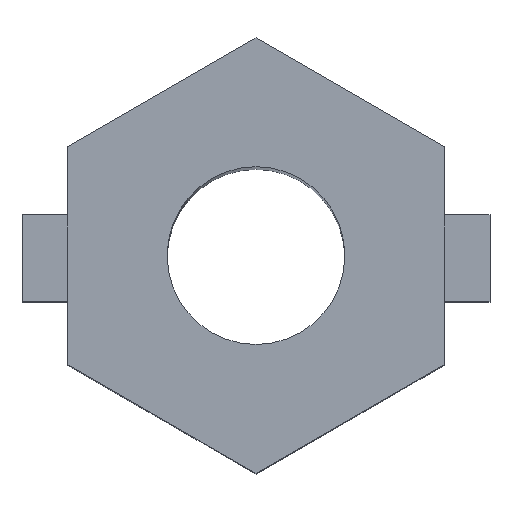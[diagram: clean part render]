
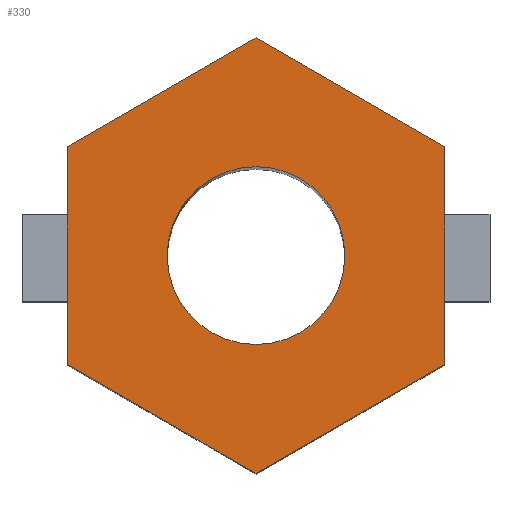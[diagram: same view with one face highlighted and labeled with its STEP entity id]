
A CAD part, top view. The second image highlights one B-rep face of the part: STEP entity #330.
In plain terms, the highlighted planar face has unit normal (0, 0, 1).
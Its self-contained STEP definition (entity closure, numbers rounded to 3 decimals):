
#1 = VERTEX_POINT ( 'NONE', #1367 ) ;
#13 = CARTESIAN_POINT ( 'NONE',  ( -23.823, 27.047, 15. ) ) ;
#52 = DIRECTION ( 'NONE',  ( 1., 0., 0. ) ) ;
#78 = CARTESIAN_POINT ( 'NONE',  ( -18.627, 30.047, 15. ) ) ;
#83 = DIRECTION ( 'NONE',  ( 0., -1., 0. ) ) ;
#88 = CIRCLE ( 'NONE', #463, 2.45 ) ;
#89 = AXIS2_PLACEMENT_3D ( 'NONE', #751, #862, #52 ) ;
#97 = ORIENTED_EDGE ( 'NONE', *, *, #455, .F. ) ;
#118 = EDGE_CURVE ( 'NONE', #213, #1092, #1169, .T. ) ;
#167 = ORIENTED_EDGE ( 'NONE', *, *, #425, .F. ) ;
#174 = CARTESIAN_POINT ( 'NONE',  ( -23.823, 27.047, 15. ) ) ;
#204 = DIRECTION ( 'NONE',  ( 0.866, 0.5, 0. ) ) ;
#213 = VERTEX_POINT ( 'NONE', #776 ) ;
#218 = VECTOR ( 'NONE', #581, 1000. ) ;
#221 = ORIENTED_EDGE ( 'NONE', *, *, #391, .F. ) ;
#222 = CARTESIAN_POINT ( 'NONE',  ( -29.02, 36.047, 15. ) ) ;
#223 = FACE_BOUND ( 'NONE', #285, .T. ) ;
#228 = CARTESIAN_POINT ( 'NONE',  ( -23.823, 39.047, 15. ) ) ;
#233 = VECTOR ( 'NONE', #83, 1000. ) ;
#237 = FACE_OUTER_BOUND ( 'NONE', #1321, .T. ) ;
#251 = ORIENTED_EDGE ( 'NONE', *, *, #569, .F. ) ;
#277 = CARTESIAN_POINT ( 'NONE',  ( -26.273, 33.047, 15. ) ) ;
#285 = EDGE_LOOP ( 'NONE', ( #353, #788 ) ) ;
#330 = ADVANCED_FACE ( 'NONE', ( #237, #223 ), #1362, .T. ) ;
#347 = LINE ( 'NONE', #13, #1227 ) ;
#353 = ORIENTED_EDGE ( 'NONE', *, *, #118, .T. ) ;
#375 = EDGE_CURVE ( 'NONE', #1092, #213, #88, .T. ) ;
#391 = EDGE_CURVE ( 'NONE', #794, #875, #1418, .T. ) ;
#425 = EDGE_CURVE ( 'NONE', #875, #1, #828, .T. ) ;
#455 = EDGE_CURVE ( 'NONE', #1, #693, #347, .T. ) ;
#463 = AXIS2_PLACEMENT_3D ( 'NONE', #731, #726, #661 ) ;
#487 = VECTOR ( 'NONE', #204, 1000. ) ;
#505 = EDGE_CURVE ( 'NONE', #693, #1348, #1429, .T. ) ;
#533 = LINE ( 'NONE', #228, #487 ) ;
#544 = EDGE_CURVE ( 'NONE', #1348, #570, #879, .T. ) ;
#545 = DIRECTION ( 'NONE',  ( 0.866, -0.5, 0. ) ) ;
#569 = EDGE_CURVE ( 'NONE', #570, #794, #533, .T. ) ;
#570 = VERTEX_POINT ( 'NONE', #222 ) ;
#581 = DIRECTION ( 'NONE',  ( 0., 1., 0. ) ) ;
#618 = CARTESIAN_POINT ( 'NONE',  ( -18.627, 36.047, 15. ) ) ;
#661 = DIRECTION ( 'NONE',  ( 1., 0., 0. ) ) ;
#693 = VERTEX_POINT ( 'NONE', #174 ) ;
#694 = CARTESIAN_POINT ( 'NONE',  ( -29.02, 36.047, 15. ) ) ;
#712 = ORIENTED_EDGE ( 'NONE', *, *, #544, .F. ) ;
#717 = CARTESIAN_POINT ( 'NONE',  ( -29.02, 30.047, 15. ) ) ;
#726 = DIRECTION ( 'NONE',  ( 0., 0., -1. ) ) ;
#731 = CARTESIAN_POINT ( 'NONE',  ( -23.823, 33.047, 15. ) ) ;
#751 = CARTESIAN_POINT ( 'NONE',  ( -23.823, 33.047, 15. ) ) ;
#776 = CARTESIAN_POINT ( 'NONE',  ( -21.373, 33.047, 15. ) ) ;
#788 = ORIENTED_EDGE ( 'NONE', *, *, #375, .T. ) ;
#793 = CARTESIAN_POINT ( 'NONE',  ( -23.823, 39.047, 15. ) ) ;
#794 = VERTEX_POINT ( 'NONE', #793 ) ;
#799 = VECTOR ( 'NONE', #545, 1000. ) ;
#828 = LINE ( 'NONE', #78, #233 ) ;
#862 = DIRECTION ( 'NONE',  ( 0., 0., -1. ) ) ;
#875 = VERTEX_POINT ( 'NONE', #1290 ) ;
#879 = LINE ( 'NONE', #694, #218 ) ;
#959 = ORIENTED_EDGE ( 'NONE', *, *, #505, .F. ) ;
#1029 = DIRECTION ( 'NONE',  ( -0.866, 0.5, 0. ) ) ;
#1032 = CARTESIAN_POINT ( 'NONE',  ( -29.02, 30.047, 15. ) ) ;
#1092 = VERTEX_POINT ( 'NONE', #277 ) ;
#1130 = VECTOR ( 'NONE', #1029, 1000. ) ;
#1169 = CIRCLE ( 'NONE', #89, 2.45 ) ;
#1227 = VECTOR ( 'NONE', #1428, 1000. ) ;
#1264 = DIRECTION ( 'NONE',  ( 1., 0., 0. ) ) ;
#1275 = DIRECTION ( 'NONE',  ( 0., 0., 1. ) ) ;
#1290 = CARTESIAN_POINT ( 'NONE',  ( -18.627, 36.047, 15. ) ) ;
#1321 = EDGE_LOOP ( 'NONE', ( #251, #712, #959, #97, #167, #221 ) ) ;
#1334 = AXIS2_PLACEMENT_3D ( 'NONE', #1380, #1275, #1264 ) ;
#1348 = VERTEX_POINT ( 'NONE', #717 ) ;
#1362 = PLANE ( 'NONE',  #1334 ) ;
#1367 = CARTESIAN_POINT ( 'NONE',  ( -18.627, 30.047, 15. ) ) ;
#1380 = CARTESIAN_POINT ( 'NONE',  ( -23.823, 33.047, 15. ) ) ;
#1418 = LINE ( 'NONE', #618, #799 ) ;
#1428 = DIRECTION ( 'NONE',  ( -0.866, -0.5, 0. ) ) ;
#1429 = LINE ( 'NONE', #1032, #1130 ) ;
